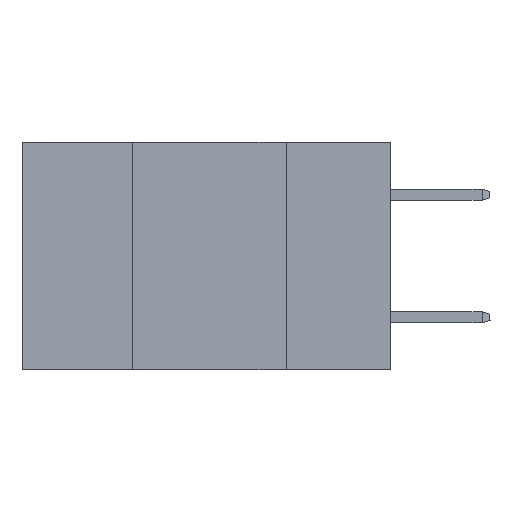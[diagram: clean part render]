
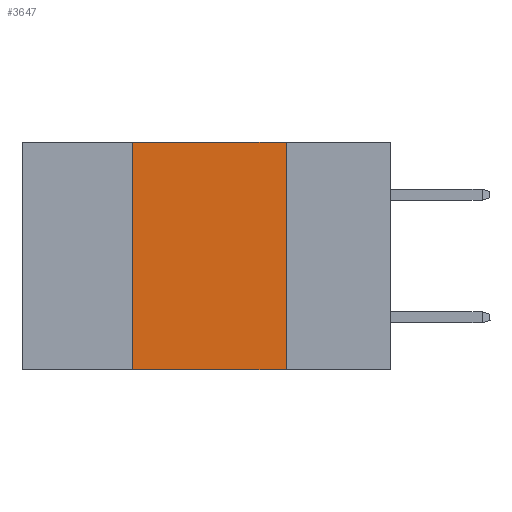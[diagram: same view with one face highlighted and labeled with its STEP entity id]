
A CAD part, left-side view. The second image highlights one B-rep face of the part: STEP entity #3647.
In plain terms, the highlighted planar face has unit normal (-1, 0, 0).
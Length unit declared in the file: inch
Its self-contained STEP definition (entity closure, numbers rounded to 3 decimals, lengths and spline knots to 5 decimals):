
#528 = DIRECTION ( 'NONE',  ( 1., 0., 0. ) ) ;
#1578 = EDGE_CURVE ( 'NONE', #18329, #14190, #12158, .T. ) ;
#1975 = DIRECTION ( 'NONE',  ( 0., 0., 1. ) ) ;
#2182 = DIRECTION ( 'NONE',  ( 0., 0., -1. ) ) ;
#2248 = LINE ( 'NONE', #18829, #18752 ) ;
#3647 = ADVANCED_FACE ( 'NONE', ( #10427 ), #8700, .F. ) ;
#3833 = VERTEX_POINT ( 'NONE', #4614 ) ;
#4521 = CARTESIAN_POINT ( 'NONE',  ( 0., 0.17, 0. ) ) ;
#4614 = CARTESIAN_POINT ( 'NONE',  ( 0., 0.17, -0.37 ) ) ;
#5431 = ORIENTED_EDGE ( 'NONE', *, *, #15033, .F. ) ;
#5698 = DIRECTION ( 'NONE',  ( 0., -1., 0. ) ) ;
#5895 = EDGE_LOOP ( 'NONE', ( #6627, #6708, #5431, #16358 ) ) ;
#6627 = ORIENTED_EDGE ( 'NONE', *, *, #9045, .F. ) ;
#6708 = ORIENTED_EDGE ( 'NONE', *, *, #1578, .F. ) ;
#7375 = VECTOR ( 'NONE', #19638, 39.37008 ) ;
#7410 = CARTESIAN_POINT ( 'NONE',  ( 0., 0.42, -0.37 ) ) ;
#7440 = VERTEX_POINT ( 'NONE', #7410 ) ;
#7761 = VECTOR ( 'NONE', #9784, 39.37008 ) ;
#8700 = PLANE ( 'NONE',  #21281 ) ;
#8774 = CARTESIAN_POINT ( 'NONE',  ( 0., 0.42, 0. ) ) ;
#9045 = EDGE_CURVE ( 'NONE', #14190, #3833, #14582, .T. ) ;
#9784 = DIRECTION ( 'NONE',  ( 0., -1., 0. ) ) ;
#10335 = VECTOR ( 'NONE', #1975, 39.37008 ) ;
#10373 = CARTESIAN_POINT ( 'NONE',  ( 0., 0.6, 0. ) ) ;
#10427 = FACE_OUTER_BOUND ( 'NONE', #5895, .T. ) ;
#10602 = LINE ( 'NONE', #8774, #10335 ) ;
#11416 = EDGE_CURVE ( 'NONE', #7440, #3833, #2248, .T. ) ;
#12158 = LINE ( 'NONE', #21284, #7761 ) ;
#14190 = VERTEX_POINT ( 'NONE', #4521 ) ;
#14582 = LINE ( 'NONE', #21313, #7375 ) ;
#15033 = EDGE_CURVE ( 'NONE', #7440, #18329, #10602, .T. ) ;
#16358 = ORIENTED_EDGE ( 'NONE', *, *, #11416, .T. ) ;
#18329 = VERTEX_POINT ( 'NONE', #19248 ) ;
#18752 = VECTOR ( 'NONE', #5698, 39.37008 ) ;
#18829 = CARTESIAN_POINT ( 'NONE',  ( 0., 0.6, -0.37 ) ) ;
#19248 = CARTESIAN_POINT ( 'NONE',  ( 0., 0.42, 0. ) ) ;
#19638 = DIRECTION ( 'NONE',  ( 0., 0., -1. ) ) ;
#21281 = AXIS2_PLACEMENT_3D ( 'NONE', #10373, #528, #2182 ) ;
#21284 = CARTESIAN_POINT ( 'NONE',  ( 0., 0.6, 0. ) ) ;
#21313 = CARTESIAN_POINT ( 'NONE',  ( 0., 0.17, 0. ) ) ;
